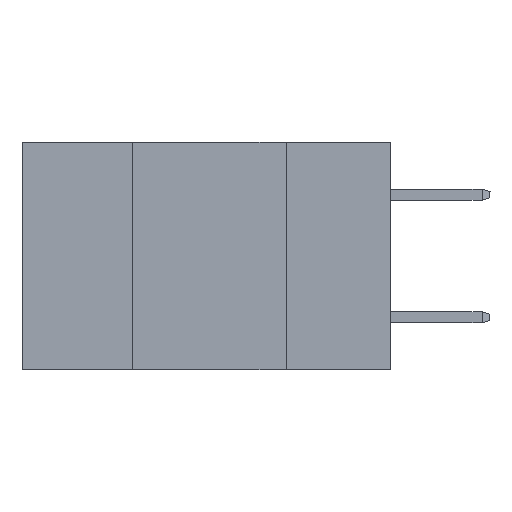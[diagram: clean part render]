
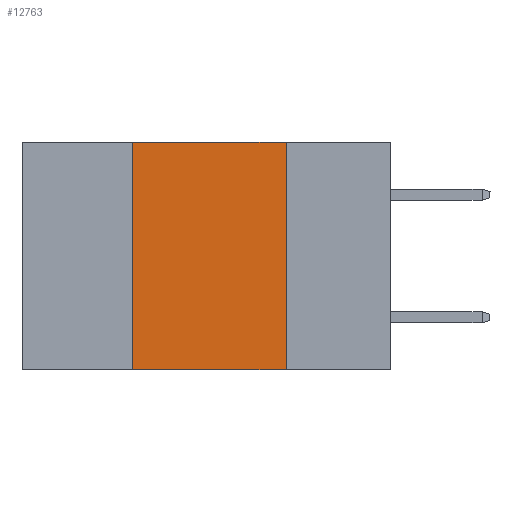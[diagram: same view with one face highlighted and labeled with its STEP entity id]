
A CAD part, left-side view. The second image highlights one B-rep face of the part: STEP entity #12763.
In plain terms, the highlighted planar face has unit normal (-1, 0, 0).
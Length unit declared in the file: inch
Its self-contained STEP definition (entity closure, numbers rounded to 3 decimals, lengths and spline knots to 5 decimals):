
#177 = CARTESIAN_POINT ( 'NONE',  ( 0., 0.17, 0. ) ) ;
#185 = VECTOR ( 'NONE', #10232, 39.37008 ) ;
#722 = DIRECTION ( 'NONE',  ( 0., -1., 0. ) ) ;
#1107 = EDGE_CURVE ( 'NONE', #11480, #7967, #7283, .T. ) ;
#1132 = EDGE_CURVE ( 'NONE', #11480, #8308, #12177, .T. ) ;
#1179 = EDGE_CURVE ( 'NONE', #8104, #7967, #2764, .T. ) ;
#2724 = CARTESIAN_POINT ( 'NONE',  ( 0., 0.6, 0. ) ) ;
#2764 = LINE ( 'NONE', #9963, #8420 ) ;
#3274 = FACE_OUTER_BOUND ( 'NONE', #5829, .T. ) ;
#3370 = EDGE_CURVE ( 'NONE', #8308, #8104, #12240, .T. ) ;
#3840 = AXIS2_PLACEMENT_3D ( 'NONE', #2724, #5126, #12530 ) ;
#4420 = CARTESIAN_POINT ( 'NONE',  ( 0., 0.42, 0. ) ) ;
#5126 = DIRECTION ( 'NONE',  ( 1., 0., 0. ) ) ;
#5829 = EDGE_LOOP ( 'NONE', ( #6413, #9572, #12335, #7125 ) ) ;
#6202 = PLANE ( 'NONE',  #3840 ) ;
#6413 = ORIENTED_EDGE ( 'NONE', *, *, #1179, .F. ) ;
#6542 = DIRECTION ( 'NONE',  ( 0., -1., 0. ) ) ;
#6672 = VECTOR ( 'NONE', #6542, 39.37008 ) ;
#6694 = CARTESIAN_POINT ( 'NONE',  ( 0., 0.6, 0. ) ) ;
#7125 = ORIENTED_EDGE ( 'NONE', *, *, #1107, .T. ) ;
#7283 = LINE ( 'NONE', #10311, #12480 ) ;
#7967 = VERTEX_POINT ( 'NONE', #9200 ) ;
#8104 = VERTEX_POINT ( 'NONE', #177 ) ;
#8308 = VERTEX_POINT ( 'NONE', #13744 ) ;
#8420 = VECTOR ( 'NONE', #9332, 39.37008 ) ;
#9200 = CARTESIAN_POINT ( 'NONE',  ( 0., 0.17, -0.37 ) ) ;
#9332 = DIRECTION ( 'NONE',  ( 0., 0., -1. ) ) ;
#9572 = ORIENTED_EDGE ( 'NONE', *, *, #3370, .F. ) ;
#9963 = CARTESIAN_POINT ( 'NONE',  ( 0., 0.17, 0. ) ) ;
#10232 = DIRECTION ( 'NONE',  ( 0., 0., 1. ) ) ;
#10311 = CARTESIAN_POINT ( 'NONE',  ( 0., 0.6, -0.37 ) ) ;
#11480 = VERTEX_POINT ( 'NONE', #13472 ) ;
#12177 = LINE ( 'NONE', #4420, #185 ) ;
#12240 = LINE ( 'NONE', #6694, #6672 ) ;
#12335 = ORIENTED_EDGE ( 'NONE', *, *, #1132, .F. ) ;
#12480 = VECTOR ( 'NONE', #722, 39.37008 ) ;
#12530 = DIRECTION ( 'NONE',  ( 0., 0., -1. ) ) ;
#12763 = ADVANCED_FACE ( 'NONE', ( #3274 ), #6202, .F. ) ;
#13472 = CARTESIAN_POINT ( 'NONE',  ( 0., 0.42, -0.37 ) ) ;
#13744 = CARTESIAN_POINT ( 'NONE',  ( 0., 0.42, 0. ) ) ;
